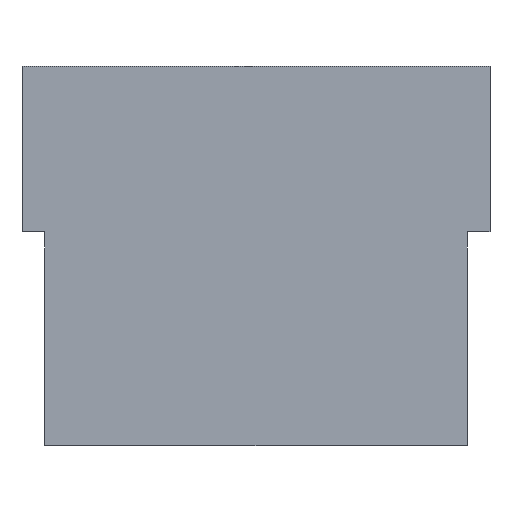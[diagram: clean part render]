
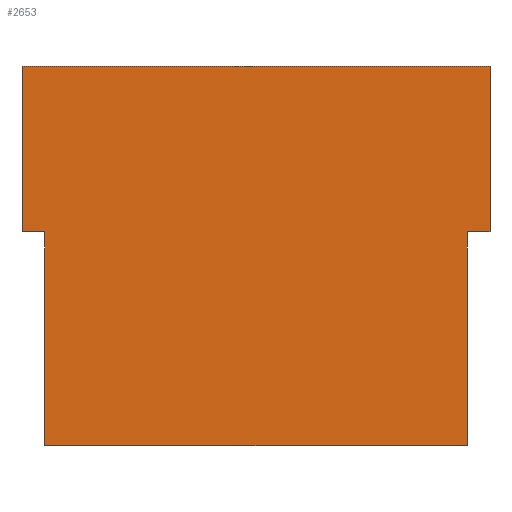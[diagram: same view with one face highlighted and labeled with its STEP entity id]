
A CAD part, front view. The second image highlights one B-rep face of the part: STEP entity #2653.
In plain terms, the highlighted planar face has unit normal (0, -1, 0).
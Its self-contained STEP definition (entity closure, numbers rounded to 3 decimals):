
#155 = DIRECTION ( 'NONE',  ( 0., 0., -1. ) ) ;
#186 = EDGE_CURVE ( 'NONE', #2794, #3440, #4130, .T. ) ;
#227 = CARTESIAN_POINT ( 'NONE',  ( 8.75, -3.15, 0.9 ) ) ;
#245 = VECTOR ( 'NONE', #5060, 1000. ) ;
#331 = CARTESIAN_POINT ( 'NONE',  ( -8.75, -3.15, 0.9 ) ) ;
#515 = CARTESIAN_POINT ( 'NONE',  ( 8.75, -3.15, 7.1 ) ) ;
#546 = VECTOR ( 'NONE', #2433, 1000. ) ;
#563 = CARTESIAN_POINT ( 'NONE',  ( -7.9, -3.15, 25.699 ) ) ;
#616 = VERTEX_POINT ( 'NONE', #4647 ) ;
#793 = AXIS2_PLACEMENT_3D ( 'NONE', #3954, #1966, #5770 ) ;
#817 = ORIENTED_EDGE ( 'NONE', *, *, #1294, .F. ) ;
#906 = ORIENTED_EDGE ( 'NONE', *, *, #4725, .F. ) ;
#1091 = LINE ( 'NONE', #515, #546 ) ;
#1294 = EDGE_CURVE ( 'NONE', #2235, #5385, #2586, .T. ) ;
#1343 = ORIENTED_EDGE ( 'NONE', *, *, #2645, .T. ) ;
#1346 = ORIENTED_EDGE ( 'NONE', *, *, #186, .F. ) ;
#1592 = LINE ( 'NONE', #4507, #2113 ) ;
#1813 = VECTOR ( 'NONE', #5225, 1000. ) ;
#1883 = CARTESIAN_POINT ( 'NONE',  ( 8.75, -3.15, 0.9 ) ) ;
#1933 = FACE_OUTER_BOUND ( 'NONE', #4924, .T. ) ;
#1966 = DIRECTION ( 'NONE',  ( 0., 1., 0. ) ) ;
#2113 = VECTOR ( 'NONE', #155, 1000. ) ;
#2235 = VERTEX_POINT ( 'NONE', #4597 ) ;
#2433 = DIRECTION ( 'NONE',  ( -1., 0., 0. ) ) ;
#2444 = DIRECTION ( 'NONE',  ( 0., 0., -1. ) ) ;
#2470 = ORIENTED_EDGE ( 'NONE', *, *, #3421, .T. ) ;
#2547 = CARTESIAN_POINT ( 'NONE',  ( 8.75, -3.15, 7.1 ) ) ;
#2586 = LINE ( 'NONE', #2643, #3338 ) ;
#2643 = CARTESIAN_POINT ( 'NONE',  ( 7.9, -3.15, 25.699 ) ) ;
#2645 = EDGE_CURVE ( 'NONE', #3142, #616, #5357, .T. ) ;
#2653 = ADVANCED_FACE ( 'NONE', ( #1933 ), #3889, .F. ) ;
#2761 = LINE ( 'NONE', #4714, #1813 ) ;
#2794 = VERTEX_POINT ( 'NONE', #2547 ) ;
#2885 = VERTEX_POINT ( 'NONE', #331 ) ;
#3138 = CARTESIAN_POINT ( 'NONE',  ( -8.75, -3.15, 7.1 ) ) ;
#3142 = VERTEX_POINT ( 'NONE', #5801 ) ;
#3225 = CARTESIAN_POINT ( 'NONE',  ( 8.75, -3.15, 7.1 ) ) ;
#3338 = VECTOR ( 'NONE', #3546, 1000. ) ;
#3355 = VERTEX_POINT ( 'NONE', #3138 ) ;
#3420 = LINE ( 'NONE', #3877, #6101 ) ;
#3421 = EDGE_CURVE ( 'NONE', #2235, #3440, #4609, .T. ) ;
#3440 = VERTEX_POINT ( 'NONE', #1883 ) ;
#3546 = DIRECTION ( 'NONE',  ( 0., 0., -1. ) ) ;
#3551 = VECTOR ( 'NONE', #2444, 1000. ) ;
#3877 = CARTESIAN_POINT ( 'NONE',  ( 8.75, -3.15, -7.1 ) ) ;
#3889 = PLANE ( 'NONE',  #793 ) ;
#3937 = DIRECTION ( 'NONE',  ( -1., 0., 0. ) ) ;
#3954 = CARTESIAN_POINT ( 'NONE',  ( 8.75, -3.15, 7.1 ) ) ;
#4130 = LINE ( 'NONE', #3225, #245 ) ;
#4261 = EDGE_CURVE ( 'NONE', #2885, #3142, #2761, .T. ) ;
#4356 = CARTESIAN_POINT ( 'NONE',  ( 7.9, -3.15, -7.1 ) ) ;
#4507 = CARTESIAN_POINT ( 'NONE',  ( -8.75, -3.15, 7.1 ) ) ;
#4597 = CARTESIAN_POINT ( 'NONE',  ( 7.9, -3.15, 0.9 ) ) ;
#4609 = LINE ( 'NONE', #227, #6271 ) ;
#4647 = CARTESIAN_POINT ( 'NONE',  ( -7.9, -3.15, -7.1 ) ) ;
#4714 = CARTESIAN_POINT ( 'NONE',  ( -7.9, -3.15, 0.9 ) ) ;
#4725 = EDGE_CURVE ( 'NONE', #5385, #616, #3420, .T. ) ;
#4924 = EDGE_LOOP ( 'NONE', ( #906, #817, #2470, #1346, #5736, #5646, #6204, #1343 ) ) ;
#5060 = DIRECTION ( 'NONE',  ( 0., 0., -1. ) ) ;
#5189 = EDGE_CURVE ( 'NONE', #3355, #2885, #1592, .T. ) ;
#5225 = DIRECTION ( 'NONE',  ( 1., 0., 0. ) ) ;
#5357 = LINE ( 'NONE', #563, #3551 ) ;
#5385 = VERTEX_POINT ( 'NONE', #4356 ) ;
#5646 = ORIENTED_EDGE ( 'NONE', *, *, #5189, .T. ) ;
#5736 = ORIENTED_EDGE ( 'NONE', *, *, #5897, .T. ) ;
#5770 = DIRECTION ( 'NONE',  ( 0., 0., 1. ) ) ;
#5801 = CARTESIAN_POINT ( 'NONE',  ( -7.9, -3.15, 0.9 ) ) ;
#5897 = EDGE_CURVE ( 'NONE', #2794, #3355, #1091, .T. ) ;
#6081 = DIRECTION ( 'NONE',  ( 1., 0., 0. ) ) ;
#6101 = VECTOR ( 'NONE', #3937, 1000. ) ;
#6204 = ORIENTED_EDGE ( 'NONE', *, *, #4261, .T. ) ;
#6271 = VECTOR ( 'NONE', #6081, 1000. ) ;
